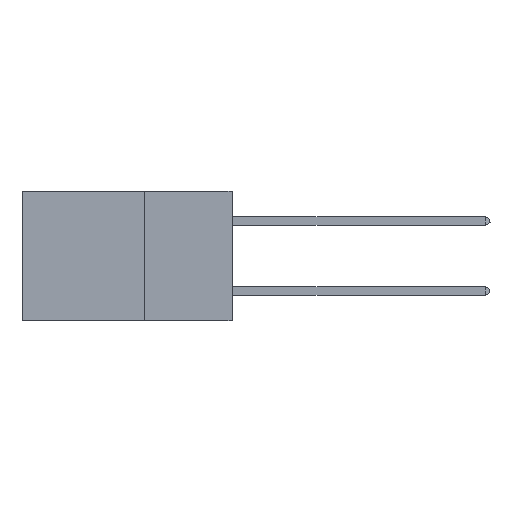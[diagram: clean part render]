
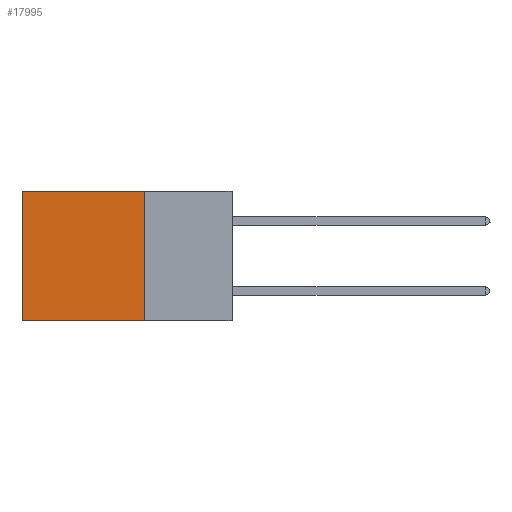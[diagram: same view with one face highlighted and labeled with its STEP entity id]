
A CAD part, left-side view. The second image highlights one B-rep face of the part: STEP entity #17995.
In plain terms, the highlighted planar face has unit normal (-1, 0, 0).
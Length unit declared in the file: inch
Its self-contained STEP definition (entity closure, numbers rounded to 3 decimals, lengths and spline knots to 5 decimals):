
#868 = DIRECTION ( 'NONE',  ( 0., 1., 0. ) ) ;
#898 = EDGE_CURVE ( 'NONE', #13139, #20402, #3885, .T. ) ;
#1073 = CARTESIAN_POINT ( 'NONE',  ( 0.2875, 0.25, 0. ) ) ;
#1098 = DIRECTION ( 'NONE',  ( 0., 0., -1. ) ) ;
#1427 = CARTESIAN_POINT ( 'NONE',  ( 0.2875, 0.25, -0.37 ) ) ;
#1673 = VERTEX_POINT ( 'NONE', #14934 ) ;
#1745 = DIRECTION ( 'NONE',  ( 0., 0., -1. ) ) ;
#3797 = VECTOR ( 'NONE', #21413, 39.37008 ) ;
#3885 = LINE ( 'NONE', #11701, #3797 ) ;
#4388 = PLANE ( 'NONE',  #21221 ) ;
#6915 = LINE ( 'NONE', #12968, #24373 ) ;
#8586 = VECTOR ( 'NONE', #1745, 39.37008 ) ;
#10710 = FACE_OUTER_BOUND ( 'NONE', #23684, .T. ) ;
#10944 = EDGE_CURVE ( 'NONE', #20402, #1673, #18319, .T. ) ;
#11701 = CARTESIAN_POINT ( 'NONE',  ( 0.2875, 0.25, 0. ) ) ;
#12606 = ORIENTED_EDGE ( 'NONE', *, *, #24809, .T. ) ;
#12968 = CARTESIAN_POINT ( 'NONE',  ( 0.2875, 0.25, 0. ) ) ;
#13139 = VERTEX_POINT ( 'NONE', #1073 ) ;
#13644 = VERTEX_POINT ( 'NONE', #23541 ) ;
#14472 = DIRECTION ( 'NONE',  ( 1., 0., 0. ) ) ;
#14872 = LINE ( 'NONE', #18933, #8586 ) ;
#14934 = CARTESIAN_POINT ( 'NONE',  ( 0.2875, 0.6, -0.37 ) ) ;
#16041 = EDGE_CURVE ( 'NONE', #13139, #13644, #6915, .T. ) ;
#17995 = ADVANCED_FACE ( 'NONE', ( #10710 ), #4388, .F. ) ;
#18181 = CARTESIAN_POINT ( 'NONE',  ( 0.2875, 0.25, -0.37 ) ) ;
#18319 = LINE ( 'NONE', #18181, #19034 ) ;
#18667 = DIRECTION ( 'NONE',  ( 0., 1., 0. ) ) ;
#18933 = CARTESIAN_POINT ( 'NONE',  ( 0.2875, 0.6, 0. ) ) ;
#19034 = VECTOR ( 'NONE', #868, 39.37008 ) ;
#19747 = ORIENTED_EDGE ( 'NONE', *, *, #898, .F. ) ;
#19794 = CARTESIAN_POINT ( 'NONE',  ( 0.2875, 0.25, 0. ) ) ;
#20402 = VERTEX_POINT ( 'NONE', #1427 ) ;
#21221 = AXIS2_PLACEMENT_3D ( 'NONE', #19794, #14472, #1098 ) ;
#21413 = DIRECTION ( 'NONE',  ( 0., 0., -1. ) ) ;
#22073 = ORIENTED_EDGE ( 'NONE', *, *, #16041, .T. ) ;
#22539 = ORIENTED_EDGE ( 'NONE', *, *, #10944, .F. ) ;
#23541 = CARTESIAN_POINT ( 'NONE',  ( 0.2875, 0.6, 0. ) ) ;
#23684 = EDGE_LOOP ( 'NONE', ( #12606, #22539, #19747, #22073 ) ) ;
#24373 = VECTOR ( 'NONE', #18667, 39.37008 ) ;
#24809 = EDGE_CURVE ( 'NONE', #13644, #1673, #14872, .T. ) ;
